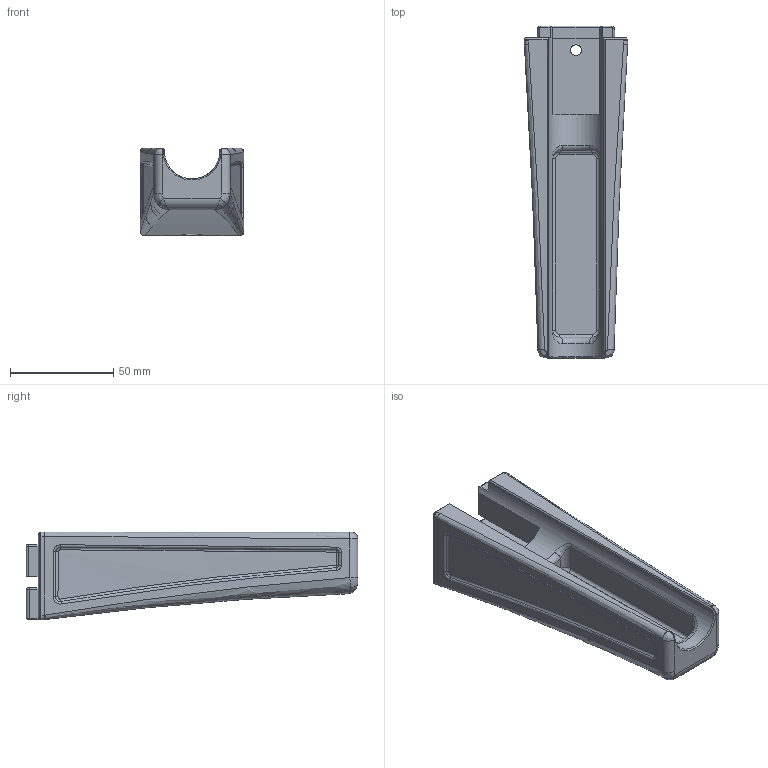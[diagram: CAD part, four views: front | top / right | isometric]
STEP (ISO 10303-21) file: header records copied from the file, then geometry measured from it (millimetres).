
FILE_DESCRIPTION(/* description */ (''),/* implementation_level */ '2;1');
FILE_NAME(/* name */ 'Chassis Forend.step',/* time_stamp */ '2021-08-06T21:53:42-04:00',/* author */ (''),/* organization */ (''),/* preprocessor_version */ 'ST-DEVELOPER v18.1',/* originating_system */ 'Autodesk Translation Framework v10.9.0.1377',/* authorisation */ '');
FILE_SCHEMA (('AUTOMOTIVE_DESIGN { 1 0 10303 214 3 1 1 }'));
Length unit declared in the file: millimetre
Products named in the file (1): Chassis Forend
Bounding box: 50.15 x 160.8 x 42.49 mm (x, y, z)
Volume: 149123.4 mm3; surface area: 33301.4 mm2
Topology: 1 solids, 1 shells, 171 faces, 414 edges, 248 vertices
Faces by surface type: bspline 77, plane 44, cylinder 41, torus 6, cone 3
Full cylindrical faces by diameter (mm): 3.8 x2, 5.3 x1, 9 x1
Entity records: 7883 total; most frequent: CARTESIAN_POINT 4342, ORIENTED_EDGE 824, DIRECTION 556, EDGE_CURVE 412, VERTEX_POINT 248, AXIS2_PLACEMENT_3D 203, EDGE_LOOP 178, FACE_OUTER_BOUND 171
